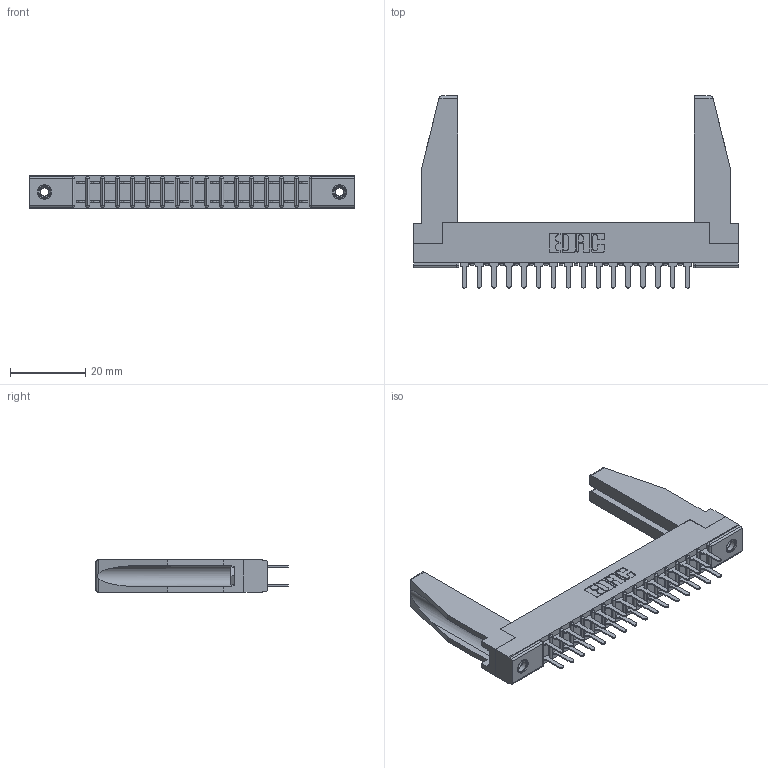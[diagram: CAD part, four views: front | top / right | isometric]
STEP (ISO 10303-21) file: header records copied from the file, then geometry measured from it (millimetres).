
FILE_DESCRIPTION (( 'STEP AP203' ), '1' );
FILE_NAME ('307-032-520-278.STEP', '2019-09-06T01:22:14', ( '' ), ( '' ), 'SwSTEP 2.0', 'SolidWorks 2016', '' );
FILE_SCHEMA (( 'CONFIG_CONTROL_DESIGN' ));
Length unit declared in the file: inch
Products named in the file (5): 307 Part_.156 Dia Mounting Holes; 345-250-001_345-250-001-102; 307-290-001_520; 307-220-078; 307-032-520-278
Assembly tree (37 placements, depth 2):
  307-032-520-278
    307 Part_.156 Dia Mounting Holes
    307-290-001_520  x32
    307-220-078  x2
    345-250-001_345-250-001-102  x2
Bounding box: 86.41 x 51.13 x 8.71 mm (x, y, z)
Volume: 9669.7 mm3; surface area: 13624.8 mm2
Topology: 37 solids, 37 shells, 1737 faces, 4813 edges, 3110 vertices
Faces by surface type: plane 1146, cylinder 541, sphere 34, cone 12, torus 4
Entity records: 19841 total; most frequent: CARTESIAN_POINT 3262, ORIENTED_EDGE 3188, DIRECTION 3160, EDGE_CURVE 1594, LINE 1216, VECTOR 1216, VERTEX_POINT 1032, AXIS2_PLACEMENT_3D 972
